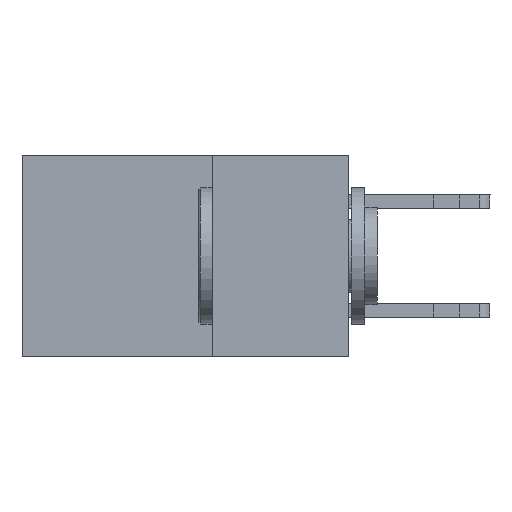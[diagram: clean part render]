
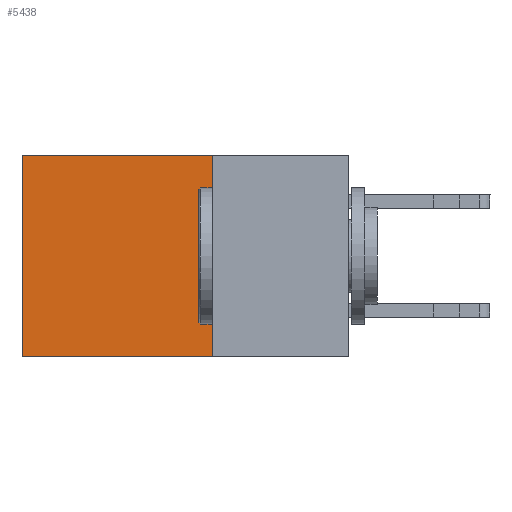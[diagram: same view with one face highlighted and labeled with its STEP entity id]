
A CAD part, left-side view. The second image highlights one B-rep face of the part: STEP entity #5438.
In plain terms, the highlighted planar face has unit normal (-1, 0, 0).
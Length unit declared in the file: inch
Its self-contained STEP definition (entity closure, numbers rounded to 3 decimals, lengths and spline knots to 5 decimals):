
#2254 = EDGE_CURVE ( 'NONE', #5889, #2297, #12619, .T. ) ;
#2297 = VERTEX_POINT ( 'NONE', #17794 ) ;
#2894 = CARTESIAN_POINT ( 'NONE',  ( 0.298, 0.25, 0. ) ) ;
#5021 = DIRECTION ( 'NONE',  ( 0., 0., -1. ) ) ;
#5438 = ADVANCED_FACE ( 'NONE', ( #10336 ), #19516, .F. ) ;
#5889 = VERTEX_POINT ( 'NONE', #10650 ) ;
#5989 = EDGE_LOOP ( 'NONE', ( #15528, #23851, #8248, #9393 ) ) ;
#7360 = EDGE_CURVE ( 'NONE', #23303, #5889, #15418, .T. ) ;
#8248 = ORIENTED_EDGE ( 'NONE', *, *, #8812, .F. ) ;
#8697 = DIRECTION ( 'NONE',  ( 0., 0., -1. ) ) ;
#8794 = CARTESIAN_POINT ( 'NONE',  ( 0.298, 0.25, 0. ) ) ;
#8812 = EDGE_CURVE ( 'NONE', #23303, #9173, #17857, .T. ) ;
#9173 = VERTEX_POINT ( 'NONE', #10486 ) ;
#9393 = ORIENTED_EDGE ( 'NONE', *, *, #7360, .T. ) ;
#10336 = FACE_OUTER_BOUND ( 'NONE', #5989, .T. ) ;
#10486 = CARTESIAN_POINT ( 'NONE',  ( 0.298, 0.25, -0.37 ) ) ;
#10650 = CARTESIAN_POINT ( 'NONE',  ( 0.298, 0.6, 0. ) ) ;
#11508 = VECTOR ( 'NONE', #8697, 39.37008 ) ;
#12118 = VECTOR ( 'NONE', #5021, 39.37008 ) ;
#12619 = LINE ( 'NONE', #16394, #11508 ) ;
#13667 = EDGE_CURVE ( 'NONE', #9173, #2297, #15888, .T. ) ;
#13927 = DIRECTION ( 'NONE',  ( 0., 1., 0. ) ) ;
#14533 = CARTESIAN_POINT ( 'NONE',  ( 0.298, 0.25, 0. ) ) ;
#15418 = LINE ( 'NONE', #23351, #22991 ) ;
#15528 = ORIENTED_EDGE ( 'NONE', *, *, #2254, .T. ) ;
#15846 = DIRECTION ( 'NONE',  ( 0., 0., -1. ) ) ;
#15888 = LINE ( 'NONE', #23104, #21799 ) ;
#16394 = CARTESIAN_POINT ( 'NONE',  ( 0.298, 0.6, 0. ) ) ;
#17794 = CARTESIAN_POINT ( 'NONE',  ( 0.298, 0.6, -0.37 ) ) ;
#17857 = LINE ( 'NONE', #8794, #12118 ) ;
#19516 = PLANE ( 'NONE',  #23107 ) ;
#21799 = VECTOR ( 'NONE', #13927, 39.37008 ) ;
#22870 = DIRECTION ( 'NONE',  ( 0., 1., 0. ) ) ;
#22991 = VECTOR ( 'NONE', #22870, 39.37008 ) ;
#23060 = DIRECTION ( 'NONE',  ( 1., 0., 0. ) ) ;
#23104 = CARTESIAN_POINT ( 'NONE',  ( 0.298, 0.25, -0.37 ) ) ;
#23107 = AXIS2_PLACEMENT_3D ( 'NONE', #2894, #23060, #15846 ) ;
#23303 = VERTEX_POINT ( 'NONE', #14533 ) ;
#23351 = CARTESIAN_POINT ( 'NONE',  ( 0.298, 0.25, 0. ) ) ;
#23851 = ORIENTED_EDGE ( 'NONE', *, *, #13667, .F. ) ;
